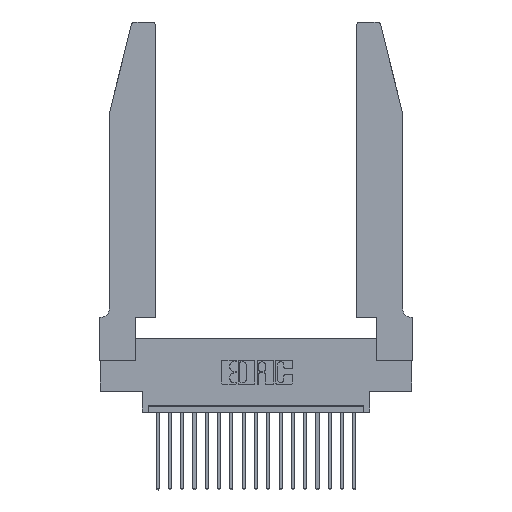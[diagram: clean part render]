
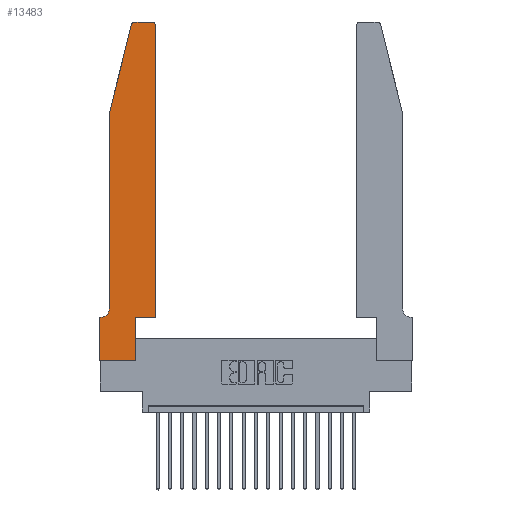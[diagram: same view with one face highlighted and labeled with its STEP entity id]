
A CAD part, top view. The second image highlights one B-rep face of the part: STEP entity #13483.
In plain terms, the highlighted planar face has unit normal (0, 0, 1).
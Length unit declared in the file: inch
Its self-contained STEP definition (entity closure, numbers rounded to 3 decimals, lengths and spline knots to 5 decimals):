
#70 = VERTEX_POINT ( 'NONE', #16136 ) ;
#135 = EDGE_CURVE ( 'NONE', #15547, #418, #20968, .T. ) ;
#418 = VERTEX_POINT ( 'NONE', #7448 ) ;
#523 = CARTESIAN_POINT ( 'NONE',  ( 0., 0.35, 0.37 ) ) ;
#599 = DIRECTION ( 'NONE',  ( 0., 0., 1. ) ) ;
#822 = CIRCLE ( 'NONE', #4982, 0.07 ) ;
#965 = VERTEX_POINT ( 'NONE', #9483 ) ;
#1024 = VECTOR ( 'NONE', #21016, 39.37008 ) ;
#1702 = CARTESIAN_POINT ( 'NONE',  ( 0.2605, 2.75, 0.37 ) ) ;
#1774 = VERTEX_POINT ( 'NONE', #6644 ) ;
#2048 = ORIENTED_EDGE ( 'NONE', *, *, #10935, .T. ) ;
#2075 = CARTESIAN_POINT ( 'NONE',  ( 0.0755, 2., 0.37 ) ) ;
#2112 = CARTESIAN_POINT ( 'NONE',  ( 0.4505, 2.72, 0.37 ) ) ;
#2383 = DIRECTION ( 'NONE',  ( 0., 0., -1. ) ) ;
#2436 = VERTEX_POINT ( 'NONE', #9847 ) ;
#2480 = ORIENTED_EDGE ( 'NONE', *, *, #11643, .T. ) ;
#2568 = ORIENTED_EDGE ( 'NONE', *, *, #8364, .T. ) ;
#2986 = CARTESIAN_POINT ( 'NONE',  ( 0.2865, 0.35, 0.37 ) ) ;
#3118 = VECTOR ( 'NONE', #6660, 39.37008 ) ;
#3187 = DIRECTION ( 'NONE',  ( 0., -1., 0. ) ) ;
#3578 = ORIENTED_EDGE ( 'NONE', *, *, #6372, .T. ) ;
#3661 = FACE_OUTER_BOUND ( 'NONE', #7619, .T. ) ;
#4097 = CARTESIAN_POINT ( 'NONE',  ( 0.0055, 0.42, 0.37 ) ) ;
#4492 = VECTOR ( 'NONE', #9019, 39.37008 ) ;
#4497 = LINE ( 'NONE', #6295, #17936 ) ;
#4982 = AXIS2_PLACEMENT_3D ( 'NONE', #4097, #2383, #10488 ) ;
#5124 = EDGE_CURVE ( 'NONE', #70, #1774, #4497, .T. ) ;
#5244 = ORIENTED_EDGE ( 'NONE', *, *, #7743, .T. ) ;
#5588 = VERTEX_POINT ( 'NONE', #6623 ) ;
#5737 = LINE ( 'NONE', #18853, #4492 ) ;
#5848 = DIRECTION ( 'NONE',  ( 0., -1., 0. ) ) ;
#6135 = VERTEX_POINT ( 'NONE', #2112 ) ;
#6253 = VERTEX_POINT ( 'NONE', #14904 ) ;
#6295 = CARTESIAN_POINT ( 'NONE',  ( 0.0755, 0.35, 0.37 ) ) ;
#6372 = EDGE_CURVE ( 'NONE', #18955, #15547, #18796, .T. ) ;
#6425 = CARTESIAN_POINT ( 'NONE',  ( 0.25487, 2.72718, 0.37 ) ) ;
#6623 = CARTESIAN_POINT ( 'NONE',  ( 0.284, 2.75, 0.37 ) ) ;
#6644 = CARTESIAN_POINT ( 'NONE',  ( 0., 0.35, 0.37 ) ) ;
#6660 = DIRECTION ( 'NONE',  ( -1., 0., 0. ) ) ;
#6975 = PLANE ( 'NONE',  #20091 ) ;
#7403 = LINE ( 'NONE', #1702, #3118 ) ;
#7448 = CARTESIAN_POINT ( 'NONE',  ( 0.4505, 0.35, 0.37 ) ) ;
#7619 = EDGE_LOOP ( 'NONE', ( #2048, #5244, #17706, #10654, #2480, #15681, #12913, #8238, #3578, #9681, #2568, #12200 ) ) ;
#7743 = EDGE_CURVE ( 'NONE', #5588, #20246, #12857, .T. ) ;
#8019 = CARTESIAN_POINT ( 'NONE',  ( 0.4505, 0.35, 0.37 ) ) ;
#8068 = EDGE_CURVE ( 'NONE', #6253, #965, #18212, .T. ) ;
#8238 = ORIENTED_EDGE ( 'NONE', *, *, #8725, .T. ) ;
#8364 = EDGE_CURVE ( 'NONE', #418, #6135, #9005, .T. ) ;
#8725 = EDGE_CURVE ( 'NONE', #2436, #18955, #5737, .T. ) ;
#8736 = CARTESIAN_POINT ( 'NONE',  ( 0.2865, 0.35, 0.37 ) ) ;
#8923 = LINE ( 'NONE', #2075, #19349 ) ;
#9005 = LINE ( 'NONE', #8019, #14080 ) ;
#9019 = DIRECTION ( 'NONE',  ( 1., 0., 0. ) ) ;
#9478 = VERTEX_POINT ( 'NONE', #17697 ) ;
#9483 = CARTESIAN_POINT ( 'NONE',  ( 0.0755, 0.42, 0.37 ) ) ;
#9681 = ORIENTED_EDGE ( 'NONE', *, *, #135, .T. ) ;
#9847 = CARTESIAN_POINT ( 'NONE',  ( 0., 0., 0.37 ) ) ;
#10048 = DIRECTION ( 'NONE',  ( -0.239, -0.971, 0. ) ) ;
#10488 = DIRECTION ( 'NONE',  ( -1., 0., 0. ) ) ;
#10654 = ORIENTED_EDGE ( 'NONE', *, *, #8068, .T. ) ;
#10935 = EDGE_CURVE ( 'NONE', #9478, #5588, #7403, .T. ) ;
#11577 = DIRECTION ( 'NONE',  ( 0., 0., 1. ) ) ;
#11643 = EDGE_CURVE ( 'NONE', #965, #70, #822, .T. ) ;
#12200 = ORIENTED_EDGE ( 'NONE', *, *, #15502, .T. ) ;
#12857 = CIRCLE ( 'NONE', #16869, 0.03 ) ;
#12913 = ORIENTED_EDGE ( 'NONE', *, *, #20470, .T. ) ;
#13483 = ADVANCED_FACE ( 'NONE', ( #3661 ), #6975, .T. ) ;
#13556 = DIRECTION ( 'NONE',  ( 1., 0., 0. ) ) ;
#14080 = VECTOR ( 'NONE', #21056, 39.37008 ) ;
#14326 = DIRECTION ( 'NONE',  ( 1., 0., 0. ) ) ;
#14562 = CARTESIAN_POINT ( 'NONE',  ( 0.0755, 2., 0.37 ) ) ;
#14904 = CARTESIAN_POINT ( 'NONE',  ( 0.0755, 2., 0.37 ) ) ;
#15502 = EDGE_CURVE ( 'NONE', #6135, #9478, #20611, .T. ) ;
#15547 = VERTEX_POINT ( 'NONE', #8736 ) ;
#15681 = ORIENTED_EDGE ( 'NONE', *, *, #5124, .T. ) ;
#15716 = AXIS2_PLACEMENT_3D ( 'NONE', #16644, #20081, #13556 ) ;
#16136 = CARTESIAN_POINT ( 'NONE',  ( 0.0055, 0.35, 0.37 ) ) ;
#16279 = DIRECTION ( 'NONE',  ( 1., 0., 0. ) ) ;
#16609 = VECTOR ( 'NONE', #16279, 39.37008 ) ;
#16644 = CARTESIAN_POINT ( 'NONE',  ( 0.4205, 2.72, 0.37 ) ) ;
#16869 = AXIS2_PLACEMENT_3D ( 'NONE', #17641, #11577, #14326 ) ;
#17126 = CARTESIAN_POINT ( 'NONE',  ( 0.2865, 0., 0.37 ) ) ;
#17204 = CARTESIAN_POINT ( 'NONE',  ( 0., 0., 0.37 ) ) ;
#17579 = DIRECTION ( 'NONE',  ( -1., 0., 0. ) ) ;
#17641 = CARTESIAN_POINT ( 'NONE',  ( 0.284, 2.72, 0.37 ) ) ;
#17697 = CARTESIAN_POINT ( 'NONE',  ( 0.4205, 2.75, 0.37 ) ) ;
#17706 = ORIENTED_EDGE ( 'NONE', *, *, #20916, .T. ) ;
#17870 = CARTESIAN_POINT ( 'NONE',  ( 0.4505, 0.35, 0.37 ) ) ;
#17936 = VECTOR ( 'NONE', #17579, 39.37008 ) ;
#18212 = LINE ( 'NONE', #14562, #19732 ) ;
#18404 = LINE ( 'NONE', #17204, #19393 ) ;
#18482 = DIRECTION ( 'NONE',  ( 1., 0., 0. ) ) ;
#18796 = LINE ( 'NONE', #2986, #1024 ) ;
#18853 = CARTESIAN_POINT ( 'NONE',  ( 0., 0., 0.37 ) ) ;
#18955 = VERTEX_POINT ( 'NONE', #17126 ) ;
#19349 = VECTOR ( 'NONE', #10048, 39.37008 ) ;
#19393 = VECTOR ( 'NONE', #5848, 39.37008 ) ;
#19732 = VECTOR ( 'NONE', #3187, 39.37008 ) ;
#20081 = DIRECTION ( 'NONE',  ( 0., 0., 1. ) ) ;
#20091 = AXIS2_PLACEMENT_3D ( 'NONE', #523, #599, #18482 ) ;
#20246 = VERTEX_POINT ( 'NONE', #6425 ) ;
#20470 = EDGE_CURVE ( 'NONE', #1774, #2436, #18404, .T. ) ;
#20611 = CIRCLE ( 'NONE', #15716, 0.03 ) ;
#20916 = EDGE_CURVE ( 'NONE', #20246, #6253, #8923, .T. ) ;
#20968 = LINE ( 'NONE', #17870, #16609 ) ;
#21016 = DIRECTION ( 'NONE',  ( 0., 1., 0. ) ) ;
#21056 = DIRECTION ( 'NONE',  ( 0., 1., 0. ) ) ;
